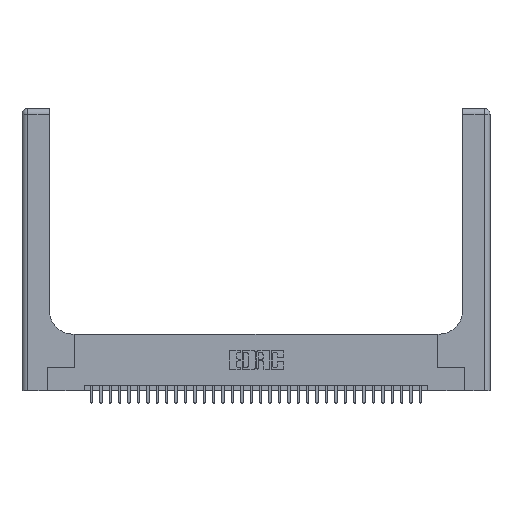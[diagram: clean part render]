
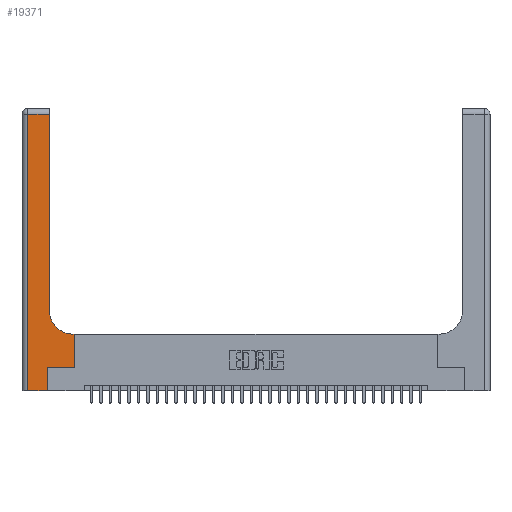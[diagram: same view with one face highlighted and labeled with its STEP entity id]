
A CAD part, top view. The second image highlights one B-rep face of the part: STEP entity #19371.
In plain terms, the highlighted planar face has unit normal (0, 0, 1).
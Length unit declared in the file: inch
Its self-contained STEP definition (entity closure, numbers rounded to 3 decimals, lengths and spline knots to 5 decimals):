
#249 = VECTOR ( 'NONE', #30408, 39.37008 ) ;
#731 = ORIENTED_EDGE ( 'NONE', *, *, #7621, .T. ) ;
#996 = DIRECTION ( 'NONE',  ( 0., 0., -1. ) ) ;
#1255 = VERTEX_POINT ( 'NONE', #28210 ) ;
#1809 = VERTEX_POINT ( 'NONE', #28057 ) ;
#4035 = LINE ( 'NONE', #17590, #22747 ) ;
#4054 = CARTESIAN_POINT ( 'NONE',  ( 0.2915, 3., 0.37 ) ) ;
#4076 = VERTEX_POINT ( 'NONE', #10952 ) ;
#4356 = DIRECTION ( 'NONE',  ( -1., 0., 0. ) ) ;
#4525 = VERTEX_POINT ( 'NONE', #28603 ) ;
#4548 = EDGE_CURVE ( 'NONE', #1255, #4525, #32825, .T. ) ;
#4822 = CIRCLE ( 'NONE', #21023, 0.25 ) ;
#5601 = DIRECTION ( 'NONE',  ( 1., 0., 0. ) ) ;
#5618 = EDGE_CURVE ( 'NONE', #33558, #1255, #7342, .T. ) ;
#6854 = VECTOR ( 'NONE', #21981, 39.37008 ) ;
#7342 = LINE ( 'NONE', #27727, #249 ) ;
#7553 = CARTESIAN_POINT ( 'NONE',  ( 0.2915, 0.6, 0.37 ) ) ;
#7621 = EDGE_CURVE ( 'NONE', #27921, #18560, #32031, .T. ) ;
#7843 = VERTEX_POINT ( 'NONE', #27476 ) ;
#9338 = LINE ( 'NONE', #4054, #20916 ) ;
#10112 = DIRECTION ( 'NONE',  ( -1., 0., 0. ) ) ;
#10123 = VECTOR ( 'NONE', #5601, 39.37008 ) ;
#10693 = CARTESIAN_POINT ( 'NONE',  ( 0.269, 0., 0.37 ) ) ;
#10952 = CARTESIAN_POINT ( 'NONE',  ( 0.269, 0.25, 0.37 ) ) ;
#11163 = CARTESIAN_POINT ( 'NONE',  ( 0., 3., 0.37 ) ) ;
#11923 = EDGE_LOOP ( 'NONE', ( #16099, #17748, #12376, #731, #12811, #16134, #31839, #12412, #21970 ) ) ;
#12023 = LINE ( 'NONE', #10693, #26069 ) ;
#12376 = ORIENTED_EDGE ( 'NONE', *, *, #17202, .T. ) ;
#12412 = ORIENTED_EDGE ( 'NONE', *, *, #4548, .T. ) ;
#12811 = ORIENTED_EDGE ( 'NONE', *, *, #23499, .T. ) ;
#13835 = DIRECTION ( 'NONE',  ( 0., 0., -1. ) ) ;
#15504 = CARTESIAN_POINT ( 'NONE',  ( 0.5585, 0.25, 0.37 ) ) ;
#15760 = AXIS2_PLACEMENT_3D ( 'NONE', #11163, #13835, #32302 ) ;
#16093 = LINE ( 'NONE', #21879, #29312 ) ;
#16099 = ORIENTED_EDGE ( 'NONE', *, *, #31578, .T. ) ;
#16134 = ORIENTED_EDGE ( 'NONE', *, *, #18763, .T. ) ;
#16609 = EDGE_CURVE ( 'NONE', #4525, #7843, #4822, .T. ) ;
#16901 = CARTESIAN_POINT ( 'NONE',  ( 0.5415, 0.85, 0.37 ) ) ;
#17202 = EDGE_CURVE ( 'NONE', #24442, #27921, #27976, .T. ) ;
#17590 = CARTESIAN_POINT ( 'NONE',  ( 0., 2.94, 0.37 ) ) ;
#17748 = ORIENTED_EDGE ( 'NONE', *, *, #18259, .T. ) ;
#18259 = EDGE_CURVE ( 'NONE', #1809, #24442, #4035, .T. ) ;
#18560 = VERTEX_POINT ( 'NONE', #26467 ) ;
#18763 = EDGE_CURVE ( 'NONE', #4076, #33558, #16093, .T. ) ;
#18821 = CARTESIAN_POINT ( 'NONE',  ( 0., 0., 0.37 ) ) ;
#19043 = PLANE ( 'NONE',  #15760 ) ;
#19371 = ADVANCED_FACE ( 'NONE', ( #20601 ), #19043, .F. ) ;
#19568 = DIRECTION ( 'NONE',  ( 1., 0., 0. ) ) ;
#20601 = FACE_OUTER_BOUND ( 'NONE', #11923, .T. ) ;
#20916 = VECTOR ( 'NONE', #25253, 39.37008 ) ;
#20947 = CARTESIAN_POINT ( 'NONE',  ( 0.06, 2.94, 0.37 ) ) ;
#21023 = AXIS2_PLACEMENT_3D ( 'NONE', #16901, #996, #19568 ) ;
#21879 = CARTESIAN_POINT ( 'NONE',  ( 0.269, 0.25, 0.37 ) ) ;
#21970 = ORIENTED_EDGE ( 'NONE', *, *, #16609, .T. ) ;
#21981 = DIRECTION ( 'NONE',  ( 0., -1., 0. ) ) ;
#22747 = VECTOR ( 'NONE', #4356, 39.37008 ) ;
#23499 = EDGE_CURVE ( 'NONE', #18560, #4076, #12023, .T. ) ;
#24442 = VERTEX_POINT ( 'NONE', #20947 ) ;
#25006 = VECTOR ( 'NONE', #10112, 39.37008 ) ;
#25152 = CARTESIAN_POINT ( 'NONE',  ( 0.06, 0., 0.37 ) ) ;
#25253 = DIRECTION ( 'NONE',  ( 0., 1., 0. ) ) ;
#26069 = VECTOR ( 'NONE', #29184, 39.37008 ) ;
#26467 = CARTESIAN_POINT ( 'NONE',  ( 0.269, 0., 0.37 ) ) ;
#27476 = CARTESIAN_POINT ( 'NONE',  ( 0.2915, 0.85, 0.37 ) ) ;
#27727 = CARTESIAN_POINT ( 'NONE',  ( 0.5585, 0.25, 0.37 ) ) ;
#27921 = VERTEX_POINT ( 'NONE', #25152 ) ;
#27976 = LINE ( 'NONE', #32445, #6854 ) ;
#28057 = CARTESIAN_POINT ( 'NONE',  ( 0.2915, 2.94, 0.37 ) ) ;
#28210 = CARTESIAN_POINT ( 'NONE',  ( 0.5585, 0.6, 0.37 ) ) ;
#28603 = CARTESIAN_POINT ( 'NONE',  ( 0.5415, 0.6, 0.37 ) ) ;
#29184 = DIRECTION ( 'NONE',  ( 0., 1., 0. ) ) ;
#29312 = VECTOR ( 'NONE', #32451, 39.37008 ) ;
#30408 = DIRECTION ( 'NONE',  ( 0., 1., 0. ) ) ;
#31578 = EDGE_CURVE ( 'NONE', #7843, #1809, #9338, .T. ) ;
#31839 = ORIENTED_EDGE ( 'NONE', *, *, #5618, .T. ) ;
#32031 = LINE ( 'NONE', #18821, #10123 ) ;
#32302 = DIRECTION ( 'NONE',  ( -1., 0., 0. ) ) ;
#32445 = CARTESIAN_POINT ( 'NONE',  ( 0.06, 3., 0.37 ) ) ;
#32451 = DIRECTION ( 'NONE',  ( 1., 0., 0. ) ) ;
#32825 = LINE ( 'NONE', #7553, #25006 ) ;
#33558 = VERTEX_POINT ( 'NONE', #15504 ) ;
